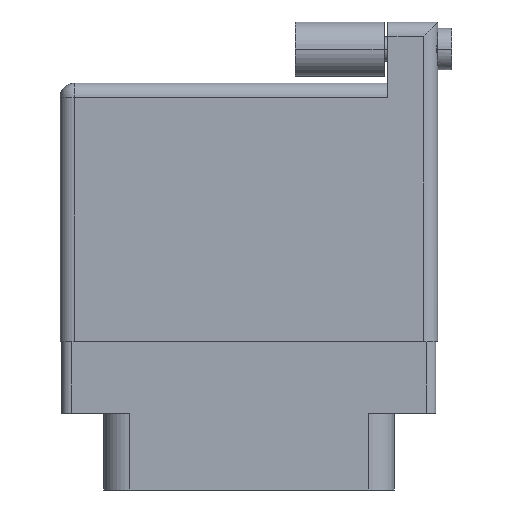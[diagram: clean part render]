
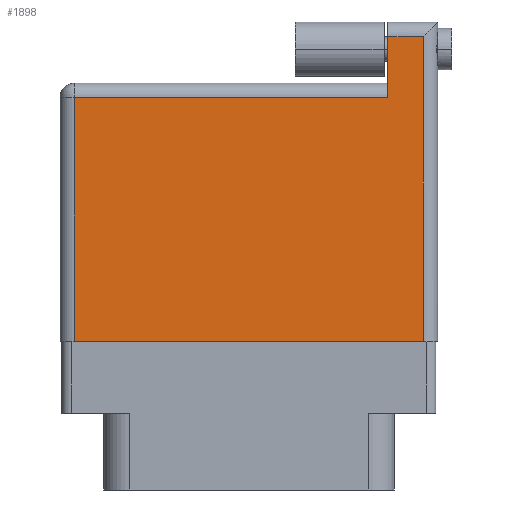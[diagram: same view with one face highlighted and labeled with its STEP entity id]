
A CAD part, front view. The second image highlights one B-rep face of the part: STEP entity #1898.
In plain terms, the highlighted face is planar.
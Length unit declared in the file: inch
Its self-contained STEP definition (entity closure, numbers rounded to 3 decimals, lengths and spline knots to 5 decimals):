
#243 = EDGE_LOOP ( 'NONE', ( #10091, #4761, #7945, #13044, #2731, #7154 ) ) ;
#564 = VERTEX_POINT ( 'NONE', #24034 ) ;
#739 = PLANE ( 'NONE',  #16111 ) ;
#1319 = CARTESIAN_POINT ( 'NONE',  ( 1.15, 1.12, 0. ) ) ;
#1636 = CARTESIAN_POINT ( 'NONE',  ( 1.15, 0.856, 0. ) ) ;
#1898 = ADVANCED_FACE ( 'NONE', ( #7535 ), #739, .F. ) ;
#2627 = LINE ( 'NONE', #6555, #19034 ) ;
#2731 = ORIENTED_EDGE ( 'NONE', *, *, #16075, .T. ) ;
#4676 = LINE ( 'NONE', #23088, #24352 ) ;
#4761 = ORIENTED_EDGE ( 'NONE', *, *, #17181, .T. ) ;
#6317 = VECTOR ( 'NONE', #8753, 39.37008 ) ;
#6334 = CARTESIAN_POINT ( 'NONE',  ( 1.15, 1.07, 0. ) ) ;
#6555 = CARTESIAN_POINT ( 'NONE',  ( 0., 0., 0. ) ) ;
#6610 = CARTESIAN_POINT ( 'NONE',  ( 0., 0.906, 0. ) ) ;
#7154 = ORIENTED_EDGE ( 'NONE', *, *, #17603, .T. ) ;
#7191 = EDGE_CURVE ( 'NONE', #14738, #22149, #13744, .T. ) ;
#7535 = FACE_OUTER_BOUND ( 'NONE', #243, .T. ) ;
#7623 = LINE ( 'NONE', #14849, #6317 ) ;
#7945 = ORIENTED_EDGE ( 'NONE', *, *, #7191, .T. ) ;
#8666 = DIRECTION ( 'NONE',  ( 0., 0., -1. ) ) ;
#8753 = DIRECTION ( 'NONE',  ( 0., -1., 0. ) ) ;
#9194 = CARTESIAN_POINT ( 'NONE',  ( 0., 1.07, 0. ) ) ;
#9533 = VECTOR ( 'NONE', #11422, 39.37008 ) ;
#9546 = CARTESIAN_POINT ( 'NONE',  ( 0.05, 0.856, 0. ) ) ;
#10091 = ORIENTED_EDGE ( 'NONE', *, *, #23182, .T. ) ;
#10734 = DIRECTION ( 'NONE',  ( -1., 0., 0. ) ) ;
#11060 = CARTESIAN_POINT ( 'NONE',  ( 1.275, 1.07, 0. ) ) ;
#11422 = DIRECTION ( 'NONE',  ( 0., -1., 0. ) ) ;
#13044 = ORIENTED_EDGE ( 'NONE', *, *, #26560, .T. ) ;
#13744 = LINE ( 'NONE', #9194, #25272 ) ;
#14086 = LINE ( 'NONE', #1319, #9533 ) ;
#14738 = VERTEX_POINT ( 'NONE', #11060 ) ;
#14849 = CARTESIAN_POINT ( 'NONE',  ( 0.05, 0., 0. ) ) ;
#15049 = DIRECTION ( 'NONE',  ( 0., 1., 0. ) ) ;
#16075 = EDGE_CURVE ( 'NONE', #18527, #24808, #17684, .T. ) ;
#16111 = AXIS2_PLACEMENT_3D ( 'NONE', #6610, #8666, #10734 ) ;
#17181 = EDGE_CURVE ( 'NONE', #24749, #14738, #4676, .T. ) ;
#17603 = EDGE_CURVE ( 'NONE', #24808, #564, #7623, .T. ) ;
#17684 = LINE ( 'NONE', #23311, #19590 ) ;
#17798 = CARTESIAN_POINT ( 'NONE',  ( 1.275, 0., 0. ) ) ;
#18527 = VERTEX_POINT ( 'NONE', #1636 ) ;
#19034 = VECTOR ( 'NONE', #20698, 39.37008 ) ;
#19313 = DIRECTION ( 'NONE',  ( -1., 0., 0. ) ) ;
#19590 = VECTOR ( 'NONE', #19313, 39.37008 ) ;
#20698 = DIRECTION ( 'NONE',  ( 1., 0., 0. ) ) ;
#22149 = VERTEX_POINT ( 'NONE', #6334 ) ;
#23088 = CARTESIAN_POINT ( 'NONE',  ( 1.275, 1.12, 0. ) ) ;
#23182 = EDGE_CURVE ( 'NONE', #564, #24749, #2627, .T. ) ;
#23311 = CARTESIAN_POINT ( 'NONE',  ( 0., 0.856, 0. ) ) ;
#23585 = DIRECTION ( 'NONE',  ( -1., 0., 0. ) ) ;
#24034 = CARTESIAN_POINT ( 'NONE',  ( 0.05, 0., 0. ) ) ;
#24352 = VECTOR ( 'NONE', #15049, 39.37008 ) ;
#24749 = VERTEX_POINT ( 'NONE', #17798 ) ;
#24808 = VERTEX_POINT ( 'NONE', #9546 ) ;
#25272 = VECTOR ( 'NONE', #23585, 39.37008 ) ;
#26560 = EDGE_CURVE ( 'NONE', #22149, #18527, #14086, .T. ) ;
